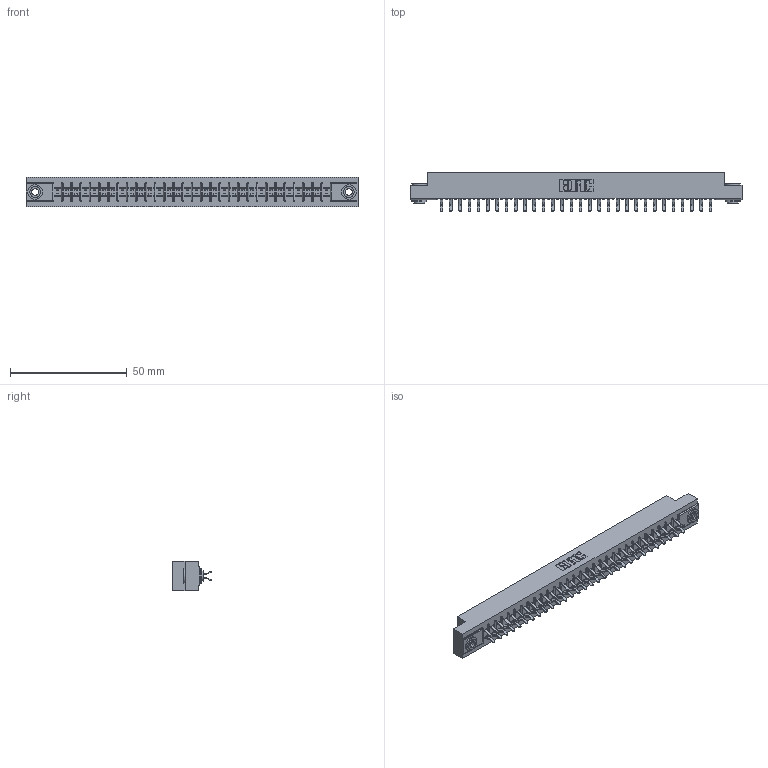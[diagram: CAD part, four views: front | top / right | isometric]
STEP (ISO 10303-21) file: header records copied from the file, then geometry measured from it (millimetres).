
FILE_DESCRIPTION (( 'STEP AP203' ), '1' );
FILE_NAME ('305-060-556-203.STEP', '2019-09-10T01:28:01', ( '' ), ( '' ), 'SwSTEP 2.0', 'SolidWorks 2016', '' );
FILE_SCHEMA (( 'CONFIG_CONTROL_DESIGN' ));
Length unit declared in the file: inch
Products named in the file (4): 345-250-002_345-250-002-102; 305 Part_.156 Dia; 305-060-556-203; 305-290-001_556
Assembly tree (63 placements, depth 2):
  305-060-556-203
    305 Part_.156 Dia
    305-290-001_556  x60
    345-250-002_345-250-002-102  x2
Bounding box: 141.88 x 16.64 x 12.7 mm (x, y, z)
Volume: 14717.9 mm3; surface area: 18727.6 mm2
Topology: 63 solids, 63 shells, 3528 faces, 10118 edges, 6580 vertices
Faces by surface type: plane 1952, cylinder 1448, sphere 120, cone 8
Entity records: 35230 total; most frequent: CARTESIAN_POINT 5813, ORIENTED_EDGE 5760, DIRECTION 5652, EDGE_CURVE 2880, VECTOR 2302, LINE 2302, VERTEX_POINT 1836, AXIS2_PLACEMENT_3D 1675
